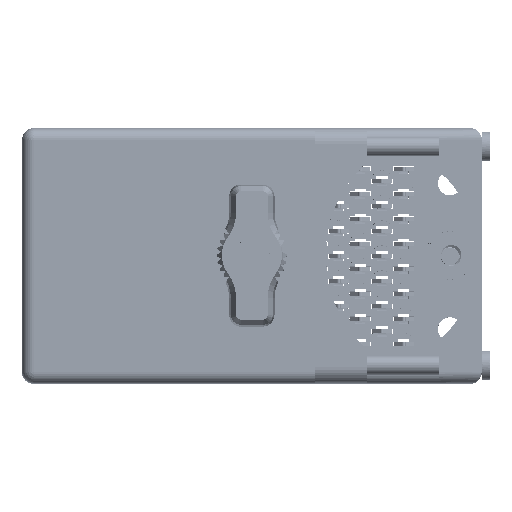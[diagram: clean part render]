
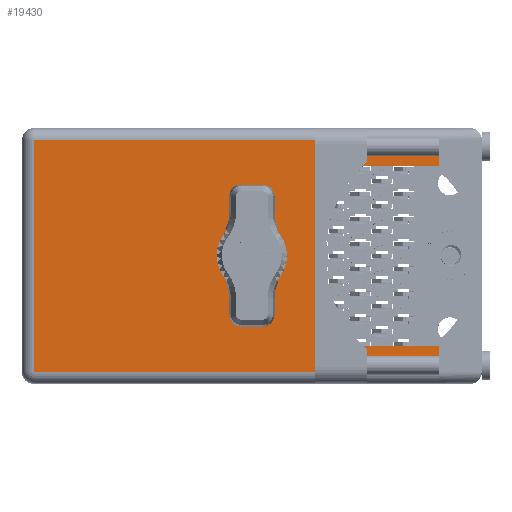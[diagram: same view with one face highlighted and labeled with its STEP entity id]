
A CAD part, top view. The second image highlights one B-rep face of the part: STEP entity #19430.
In plain terms, the highlighted face is planar.
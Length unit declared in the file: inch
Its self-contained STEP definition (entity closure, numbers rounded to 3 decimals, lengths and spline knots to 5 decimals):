
#1804 = EDGE_CURVE ( 'NONE', #35076, #80941, #56602, .T. ) ;
#1847 = CARTESIAN_POINT ( 'NONE',  ( 0., 1.93, 0. ) ) ;
#2804 = EDGE_CURVE ( 'NONE', #112684, #79997, #7075, .T. ) ;
#5246 = VERTEX_POINT ( 'NONE', #14534 ) ;
#6060 = CIRCLE ( 'NONE', #7491, 0.17 ) ;
#6516 = VERTEX_POINT ( 'NONE', #10604 ) ;
#7075 = LINE ( 'NONE', #50301, #83856 ) ;
#7147 = DIRECTION ( 'NONE',  ( 0., 0., 1. ) ) ;
#7491 = AXIS2_PLACEMENT_3D ( 'NONE', #1847, #100588, #73999 ) ;
#7524 = VECTOR ( 'NONE', #66493, 39.37008 ) ;
#7589 = VERTEX_POINT ( 'NONE', #25773 ) ;
#8418 = CARTESIAN_POINT ( 'NONE',  ( -1.3775, 1.93, -0.765 ) ) ;
#8517 = EDGE_CURVE ( 'NONE', #46388, #10359, #74569, .T. ) ;
#8811 = ORIENTED_EDGE ( 'NONE', *, *, #8517, .T. ) ;
#10359 = VERTEX_POINT ( 'NONE', #30327 ) ;
#10604 = CARTESIAN_POINT ( 'NONE',  ( 1.1215, 1.93, 0.695 ) ) ;
#11032 = ORIENTED_EDGE ( 'NONE', *, *, #77415, .T. ) ;
#11689 = VECTOR ( 'NONE', #88481, 39.37008 ) ;
#12187 = VECTOR ( 'NONE', #113434, 39.37008 ) ;
#12803 = ORIENTED_EDGE ( 'NONE', *, *, #76689, .T. ) ;
#14534 = CARTESIAN_POINT ( 'NONE',  ( 1.1215, 1.93, -0.54 ) ) ;
#14801 = LINE ( 'NONE', #75150, #87453 ) ;
#16983 = ORIENTED_EDGE ( 'NONE', *, *, #80739, .F. ) ;
#17567 = DIRECTION ( 'NONE',  ( 0., 0., -1. ) ) ;
#19430 = ADVANCED_FACE ( 'NONE', ( #46875, #37023 ), #26708, .T. ) ;
#22011 = ORIENTED_EDGE ( 'NONE', *, *, #22328, .F. ) ;
#22328 = EDGE_CURVE ( 'NONE', #112684, #6516, #14801, .T. ) ;
#25773 = CARTESIAN_POINT ( 'NONE',  ( 1.1215, 1.93, -0.695 ) ) ;
#26708 = PLANE ( 'NONE',  #74609 ) ;
#28919 = LINE ( 'NONE', #54243, #45682 ) ;
#30327 = CARTESIAN_POINT ( 'NONE',  ( -1.3075, 1.93, 0.695 ) ) ;
#35076 = VERTEX_POINT ( 'NONE', #75216 ) ;
#35209 = EDGE_LOOP ( 'NONE', ( #8811, #80380, #22011, #63031, #11032, #112402, #38439, #12803 ) ) ;
#37023 = FACE_BOUND ( 'NONE', #106365, .T. ) ;
#38439 = ORIENTED_EDGE ( 'NONE', *, *, #46929, .F. ) ;
#40496 = CARTESIAN_POINT ( 'NONE',  ( 0.4075, 1.93, -0.54 ) ) ;
#45682 = VECTOR ( 'NONE', #115519, 39.37008 ) ;
#46388 = VERTEX_POINT ( 'NONE', #58636 ) ;
#46875 = FACE_OUTER_BOUND ( 'NONE', #35209, .T. ) ;
#46929 = EDGE_CURVE ( 'NONE', #7589, #5246, #28919, .T. ) ;
#48268 = DIRECTION ( 'NONE',  ( 0., 0., 1. ) ) ;
#49237 = EDGE_CURVE ( 'NONE', #52662, #5246, #70349, .T. ) ;
#49852 = VECTOR ( 'NONE', #17567, 39.37008 ) ;
#50301 = CARTESIAN_POINT ( 'NONE',  ( 1.1215, 1.93, 0.54 ) ) ;
#50310 = ORIENTED_EDGE ( 'NONE', *, *, #1804, .F. ) ;
#52096 = DIRECTION ( 'NONE',  ( 0., 1., 0. ) ) ;
#52662 = VERTEX_POINT ( 'NONE', #40496 ) ;
#54243 = CARTESIAN_POINT ( 'NONE',  ( 1.1215, 1.93, -0.765 ) ) ;
#56602 = CIRCLE ( 'NONE', #111685, 0.17 ) ;
#58636 = CARTESIAN_POINT ( 'NONE',  ( -1.3075, 1.93, -0.695 ) ) ;
#59603 = VECTOR ( 'NONE', #104908, 39.37008 ) ;
#60068 = CARTESIAN_POINT ( 'NONE',  ( 1.1215, 1.93, 0.695 ) ) ;
#61522 = CARTESIAN_POINT ( 'NONE',  ( -1.3075, 1.93, -0.765 ) ) ;
#63031 = ORIENTED_EDGE ( 'NONE', *, *, #2804, .T. ) ;
#65116 = LINE ( 'NONE', #60068, #59603 ) ;
#65131 = LINE ( 'NONE', #106252, #49852 ) ;
#66493 = DIRECTION ( 'NONE',  ( 1., 0., 0. ) ) ;
#68911 = CARTESIAN_POINT ( 'NONE',  ( -1.3775, 1.93, -0.695 ) ) ;
#69380 = DIRECTION ( 'NONE',  ( -1., 0., 0. ) ) ;
#70349 = LINE ( 'NONE', #73884, #7524 ) ;
#71598 = DIRECTION ( 'NONE',  ( 0., 1., 0. ) ) ;
#73884 = CARTESIAN_POINT ( 'NONE',  ( 1.1215, 1.93, -0.54 ) ) ;
#73999 = DIRECTION ( 'NONE',  ( 0., 0., 1. ) ) ;
#74569 = LINE ( 'NONE', #61522, #11689 ) ;
#74609 = AXIS2_PLACEMENT_3D ( 'NONE', #8418, #71598, #89264 ) ;
#75150 = CARTESIAN_POINT ( 'NONE',  ( 1.1215, 1.93, -0.765 ) ) ;
#75216 = CARTESIAN_POINT ( 'NONE',  ( 0., 1.93, -0.17 ) ) ;
#76689 = EDGE_CURVE ( 'NONE', #7589, #46388, #80691, .T. ) ;
#77415 = EDGE_CURVE ( 'NONE', #79997, #52662, #65131, .T. ) ;
#78574 = CARTESIAN_POINT ( 'NONE',  ( 0., 1.93, 0. ) ) ;
#79997 = VERTEX_POINT ( 'NONE', #92754 ) ;
#80380 = ORIENTED_EDGE ( 'NONE', *, *, #100359, .T. ) ;
#80691 = LINE ( 'NONE', #68911, #12187 ) ;
#80739 = EDGE_CURVE ( 'NONE', #80941, #35076, #6060, .T. ) ;
#80941 = VERTEX_POINT ( 'NONE', #111163 ) ;
#83856 = VECTOR ( 'NONE', #69380, 39.37008 ) ;
#87453 = VECTOR ( 'NONE', #48268, 39.37008 ) ;
#88481 = DIRECTION ( 'NONE',  ( 0., 0., 1. ) ) ;
#89264 = DIRECTION ( 'NONE',  ( -1., 0., 0. ) ) ;
#92754 = CARTESIAN_POINT ( 'NONE',  ( 0.4075, 1.93, 0.54 ) ) ;
#100359 = EDGE_CURVE ( 'NONE', #10359, #6516, #65116, .T. ) ;
#100588 = DIRECTION ( 'NONE',  ( 0., 1., 0. ) ) ;
#104908 = DIRECTION ( 'NONE',  ( 1., 0., 0. ) ) ;
#106252 = CARTESIAN_POINT ( 'NONE',  ( 0.4075, 1.93, -0.54 ) ) ;
#106365 = EDGE_LOOP ( 'NONE', ( #16983, #50310 ) ) ;
#110902 = CARTESIAN_POINT ( 'NONE',  ( 1.1215, 1.93, 0.54 ) ) ;
#111163 = CARTESIAN_POINT ( 'NONE',  ( 0., 1.93, 0.17 ) ) ;
#111685 = AXIS2_PLACEMENT_3D ( 'NONE', #78574, #52096, #7147 ) ;
#112402 = ORIENTED_EDGE ( 'NONE', *, *, #49237, .T. ) ;
#112684 = VERTEX_POINT ( 'NONE', #110902 ) ;
#113434 = DIRECTION ( 'NONE',  ( -1., 0., 0. ) ) ;
#115519 = DIRECTION ( 'NONE',  ( 0., 0., 1. ) ) ;
